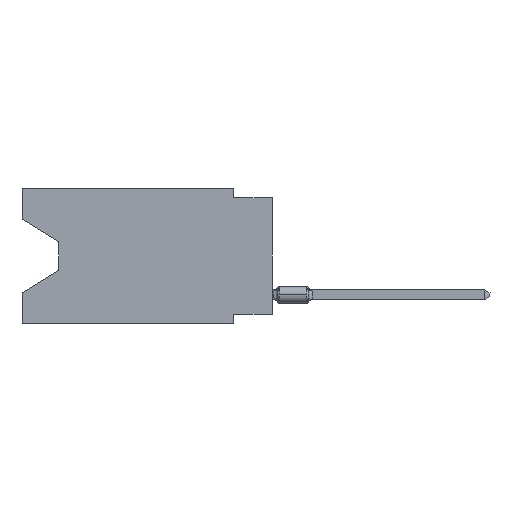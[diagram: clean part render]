
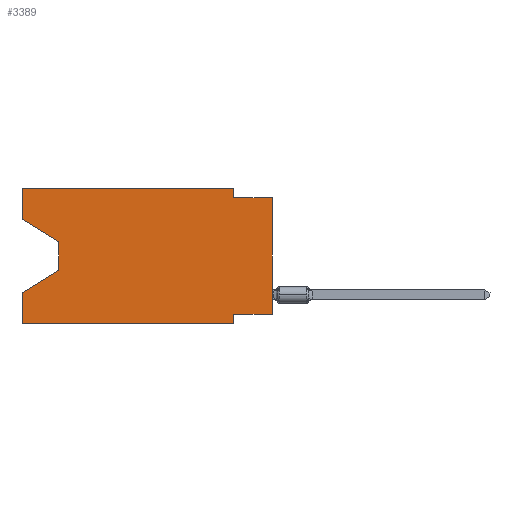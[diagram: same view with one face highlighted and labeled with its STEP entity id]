
A CAD part, left-side view. The second image highlights one B-rep face of the part: STEP entity #3389.
In plain terms, the highlighted planar face has unit normal (-1, 0, 0).
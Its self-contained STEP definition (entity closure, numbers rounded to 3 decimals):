
#610 = CARTESIAN_POINT ( 'NONE',  ( 0., 2.54, 0. ) ) ;
#782 = LINE ( 'NONE', #3093, #22673 ) ;
#973 = ORIENTED_EDGE ( 'NONE', *, *, #13961, .F. ) ;
#1056 = CARTESIAN_POINT ( 'NONE',  ( 0., 13.97, -5.385 ) ) ;
#1363 = FACE_OUTER_BOUND ( 'NONE', #5661, .T. ) ;
#1489 = VECTOR ( 'NONE', #24870, 1000. ) ;
#1556 = VECTOR ( 'NONE', #5806, 1000. ) ;
#1592 = VERTEX_POINT ( 'NONE', #11660 ) ;
#1625 = VERTEX_POINT ( 'NONE', #7302 ) ;
#1802 = CARTESIAN_POINT ( 'NONE',  ( 0., 16.383, -2.038 ) ) ;
#1903 = DIRECTION ( 'NONE',  ( 0., -1., 0. ) ) ;
#2031 = LINE ( 'NONE', #4222, #16066 ) ;
#2408 = ORIENTED_EDGE ( 'NONE', *, *, #4348, .T. ) ;
#2654 = CARTESIAN_POINT ( 'NONE',  ( 0., 2.54, -8.89 ) ) ;
#2872 = LINE ( 'NONE', #11108, #15483 ) ;
#2917 = LINE ( 'NONE', #10774, #15615 ) ;
#3093 = CARTESIAN_POINT ( 'NONE',  ( 0., 0., -8.255 ) ) ;
#3310 = DIRECTION ( 'NONE',  ( 0., 0., -1. ) ) ;
#3389 = ADVANCED_FACE ( 'NONE', ( #1363 ), #16724, .F. ) ;
#4143 = ORIENTED_EDGE ( 'NONE', *, *, #6285, .T. ) ;
#4205 = EDGE_CURVE ( 'NONE', #14072, #18288, #2872, .T. ) ;
#4222 = CARTESIAN_POINT ( 'NONE',  ( 0., 0., -0.635 ) ) ;
#4272 = VECTOR ( 'NONE', #14614, 1000. ) ;
#4348 = EDGE_CURVE ( 'NONE', #19978, #5971, #11345, .T. ) ;
#4804 = LINE ( 'NONE', #10612, #4272 ) ;
#5641 = ORIENTED_EDGE ( 'NONE', *, *, #9624, .F. ) ;
#5661 = EDGE_LOOP ( 'NONE', ( #2408, #21448, #11588, #6281, #4143, #6156, #21135, #25302, #17475, #5641, #973, #20972 ) ) ;
#5806 = DIRECTION ( 'NONE',  ( 0., -1., 0. ) ) ;
#5858 = CARTESIAN_POINT ( 'NONE',  ( 0., 16.383, 0. ) ) ;
#5971 = VERTEX_POINT ( 'NONE', #8698 ) ;
#6156 = ORIENTED_EDGE ( 'NONE', *, *, #7081, .F. ) ;
#6281 = ORIENTED_EDGE ( 'NONE', *, *, #23197, .F. ) ;
#6285 = EDGE_CURVE ( 'NONE', #8121, #9975, #11612, .T. ) ;
#7081 = EDGE_CURVE ( 'NONE', #1625, #9975, #4804, .T. ) ;
#7200 = VERTEX_POINT ( 'NONE', #1056 ) ;
#7302 = CARTESIAN_POINT ( 'NONE',  ( 0., 2.54, -8.255 ) ) ;
#7510 = LINE ( 'NONE', #13438, #13791 ) ;
#8054 = VECTOR ( 'NONE', #12963, 1000. ) ;
#8121 = VERTEX_POINT ( 'NONE', #22751 ) ;
#8647 = DIRECTION ( 'NONE',  ( 0., 1., 0. ) ) ;
#8698 = CARTESIAN_POINT ( 'NONE',  ( 0., 13.97, -3.505 ) ) ;
#8991 = DIRECTION ( 'NONE',  ( 0., 0., -1. ) ) ;
#9183 = EDGE_CURVE ( 'NONE', #14072, #1625, #782, .T. ) ;
#9624 = EDGE_CURVE ( 'NONE', #14141, #13884, #12601, .T. ) ;
#9945 = CARTESIAN_POINT ( 'NONE',  ( 0., 0., -8.255 ) ) ;
#9975 = VERTEX_POINT ( 'NONE', #2654 ) ;
#10612 = CARTESIAN_POINT ( 'NONE',  ( 0., 2.54, -8.89 ) ) ;
#10774 = CARTESIAN_POINT ( 'NONE',  ( 0., 13.97, -5.385 ) ) ;
#11108 = CARTESIAN_POINT ( 'NONE',  ( 0., 0., 0. ) ) ;
#11158 = CARTESIAN_POINT ( 'NONE',  ( 0., 13.97, -3.505 ) ) ;
#11345 = LINE ( 'NONE', #1802, #1489 ) ;
#11533 = CARTESIAN_POINT ( 'NONE',  ( 0., 16.383, -6.852 ) ) ;
#11588 = ORIENTED_EDGE ( 'NONE', *, *, #18930, .T. ) ;
#11612 = LINE ( 'NONE', #14067, #1556 ) ;
#11660 = CARTESIAN_POINT ( 'NONE',  ( 0., 16.383, 0. ) ) ;
#12309 = CARTESIAN_POINT ( 'NONE',  ( 0., 16.383, 0. ) ) ;
#12322 = VERTEX_POINT ( 'NONE', #11533 ) ;
#12349 = EDGE_CURVE ( 'NONE', #19978, #1592, #15536, .T. ) ;
#12601 = LINE ( 'NONE', #610, #21855 ) ;
#12963 = DIRECTION ( 'NONE',  ( 0., 0., -1. ) ) ;
#12972 = CARTESIAN_POINT ( 'NONE',  ( 0., 16.383, 0. ) ) ;
#13438 = CARTESIAN_POINT ( 'NONE',  ( 0., 16.383, 0. ) ) ;
#13791 = VECTOR ( 'NONE', #17426, 1000. ) ;
#13884 = VERTEX_POINT ( 'NONE', #14885 ) ;
#13961 = EDGE_CURVE ( 'NONE', #1592, #14141, #7510, .T. ) ;
#14067 = CARTESIAN_POINT ( 'NONE',  ( 0., 16.383, -8.89 ) ) ;
#14072 = VERTEX_POINT ( 'NONE', #9945 ) ;
#14141 = VERTEX_POINT ( 'NONE', #16134 ) ;
#14418 = VECTOR ( 'NONE', #24281, 1000. ) ;
#14614 = DIRECTION ( 'NONE',  ( 0., 0., -1. ) ) ;
#14885 = CARTESIAN_POINT ( 'NONE',  ( 0., 2.54, -0.635 ) ) ;
#15483 = VECTOR ( 'NONE', #20646, 1000. ) ;
#15536 = LINE ( 'NONE', #5858, #23694 ) ;
#15580 = CARTESIAN_POINT ( 'NONE',  ( 0., 16.383, -2.038 ) ) ;
#15615 = VECTOR ( 'NONE', #18636, 1000. ) ;
#16066 = VECTOR ( 'NONE', #1903, 1000. ) ;
#16134 = CARTESIAN_POINT ( 'NONE',  ( 0., 2.54, 0. ) ) ;
#16451 = LINE ( 'NONE', #12309, #14418 ) ;
#16724 = PLANE ( 'NONE',  #19241 ) ;
#17426 = DIRECTION ( 'NONE',  ( 0., -1., 0. ) ) ;
#17475 = ORIENTED_EDGE ( 'NONE', *, *, #22646, .F. ) ;
#17535 = EDGE_CURVE ( 'NONE', #5971, #7200, #20940, .T. ) ;
#18288 = VERTEX_POINT ( 'NONE', #20633 ) ;
#18636 = DIRECTION ( 'NONE',  ( 0., 0.855, -0.519 ) ) ;
#18930 = EDGE_CURVE ( 'NONE', #7200, #12322, #2917, .T. ) ;
#19241 = AXIS2_PLACEMENT_3D ( 'NONE', #12972, #22867, #3310 ) ;
#19768 = DIRECTION ( 'NONE',  ( 0., 0., 1. ) ) ;
#19978 = VERTEX_POINT ( 'NONE', #15580 ) ;
#20633 = CARTESIAN_POINT ( 'NONE',  ( 0., 0., -0.635 ) ) ;
#20646 = DIRECTION ( 'NONE',  ( 0., 0., 1. ) ) ;
#20940 = LINE ( 'NONE', #11158, #8054 ) ;
#20972 = ORIENTED_EDGE ( 'NONE', *, *, #12349, .F. ) ;
#21135 = ORIENTED_EDGE ( 'NONE', *, *, #9183, .F. ) ;
#21448 = ORIENTED_EDGE ( 'NONE', *, *, #17535, .T. ) ;
#21855 = VECTOR ( 'NONE', #8991, 1000. ) ;
#22646 = EDGE_CURVE ( 'NONE', #13884, #18288, #2031, .T. ) ;
#22673 = VECTOR ( 'NONE', #8647, 1000. ) ;
#22751 = CARTESIAN_POINT ( 'NONE',  ( 0., 16.383, -8.89 ) ) ;
#22867 = DIRECTION ( 'NONE',  ( 1., 0., 0. ) ) ;
#23197 = EDGE_CURVE ( 'NONE', #8121, #12322, #16451, .T. ) ;
#23694 = VECTOR ( 'NONE', #19768, 1000. ) ;
#24281 = DIRECTION ( 'NONE',  ( 0., 0., 1. ) ) ;
#24870 = DIRECTION ( 'NONE',  ( 0., -0.855, -0.519 ) ) ;
#25302 = ORIENTED_EDGE ( 'NONE', *, *, #4205, .T. ) ;
